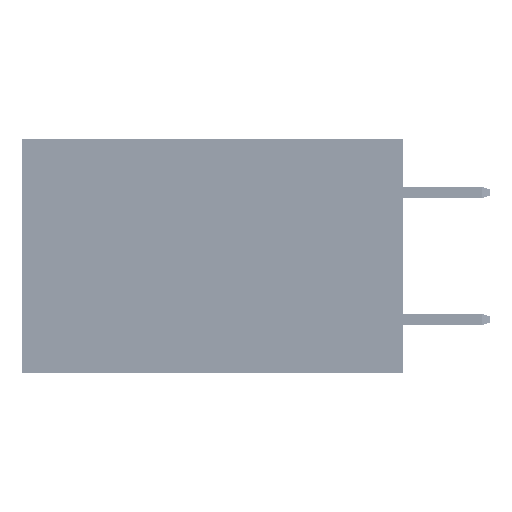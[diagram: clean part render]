
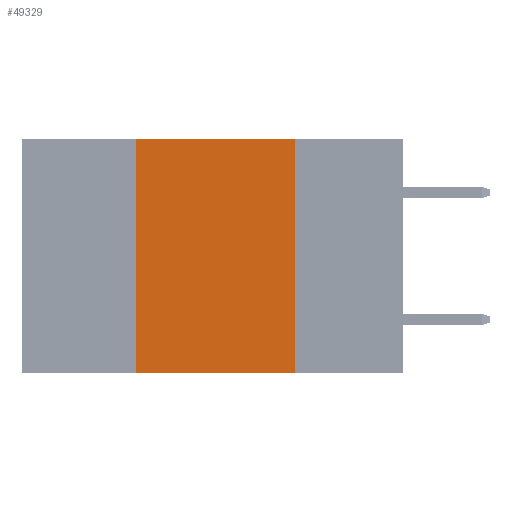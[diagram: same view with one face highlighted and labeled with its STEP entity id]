
A CAD part, left-side view. The second image highlights one B-rep face of the part: STEP entity #49329.
In plain terms, the highlighted planar face has unit normal (-1, 0, 0).
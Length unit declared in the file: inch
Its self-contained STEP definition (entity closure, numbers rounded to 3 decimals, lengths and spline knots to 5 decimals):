
#8373 = CARTESIAN_POINT ( 'NONE',  ( 0., 0.42, -0.37 ) ) ;
#9885 = ORIENTED_EDGE ( 'NONE', *, *, #15686, .F. ) ;
#10452 = DIRECTION ( 'NONE',  ( 0., 0., -1. ) ) ;
#10727 = VECTOR ( 'NONE', #41330, 39.37008 ) ;
#10737 = VERTEX_POINT ( 'NONE', #44114 ) ;
#11090 = VECTOR ( 'NONE', #43198, 39.37008 ) ;
#11476 = LINE ( 'NONE', #27892, #10727 ) ;
#12933 = PLANE ( 'NONE',  #31094 ) ;
#13321 = EDGE_LOOP ( 'NONE', ( #42781, #47987, #9885, #37089 ) ) ;
#15686 = EDGE_CURVE ( 'NONE', #40103, #10737, #46551, .T. ) ;
#16985 = CARTESIAN_POINT ( 'NONE',  ( 0., 0.6, 0. ) ) ;
#18684 = LINE ( 'NONE', #46978, #11090 ) ;
#22291 = DIRECTION ( 'NONE',  ( 0., 0., 1. ) ) ;
#22766 = CARTESIAN_POINT ( 'NONE',  ( 0., 0.17, 0. ) ) ;
#23977 = DIRECTION ( 'NONE',  ( 1., 0., 0. ) ) ;
#24784 = FACE_OUTER_BOUND ( 'NONE', #13321, .T. ) ;
#27892 = CARTESIAN_POINT ( 'NONE',  ( 0., 0.6, 0. ) ) ;
#28918 = EDGE_CURVE ( 'NONE', #40103, #43686, #18684, .T. ) ;
#30377 = CARTESIAN_POINT ( 'NONE',  ( 0., 0.42, 0. ) ) ;
#31094 = AXIS2_PLACEMENT_3D ( 'NONE', #16985, #23977, #48785 ) ;
#34374 = CARTESIAN_POINT ( 'NONE',  ( 0., 0.17, -0.37 ) ) ;
#37089 = ORIENTED_EDGE ( 'NONE', *, *, #28918, .T. ) ;
#37757 = EDGE_CURVE ( 'NONE', #10737, #52507, #11476, .T. ) ;
#37998 = VECTOR ( 'NONE', #22291, 39.37008 ) ;
#39527 = CARTESIAN_POINT ( 'NONE',  ( 0., 0.17, 0. ) ) ;
#40103 = VERTEX_POINT ( 'NONE', #8373 ) ;
#41330 = DIRECTION ( 'NONE',  ( 0., -1., 0. ) ) ;
#42781 = ORIENTED_EDGE ( 'NONE', *, *, #48281, .F. ) ;
#43198 = DIRECTION ( 'NONE',  ( 0., -1., 0. ) ) ;
#43589 = LINE ( 'NONE', #39527, #49992 ) ;
#43686 = VERTEX_POINT ( 'NONE', #34374 ) ;
#44114 = CARTESIAN_POINT ( 'NONE',  ( 0., 0.42, 0. ) ) ;
#46551 = LINE ( 'NONE', #30377, #37998 ) ;
#46978 = CARTESIAN_POINT ( 'NONE',  ( 0., 0.6, -0.37 ) ) ;
#47987 = ORIENTED_EDGE ( 'NONE', *, *, #37757, .F. ) ;
#48281 = EDGE_CURVE ( 'NONE', #52507, #43686, #43589, .T. ) ;
#48785 = DIRECTION ( 'NONE',  ( 0., 0., -1. ) ) ;
#49329 = ADVANCED_FACE ( 'NONE', ( #24784 ), #12933, .F. ) ;
#49992 = VECTOR ( 'NONE', #10452, 39.37008 ) ;
#52507 = VERTEX_POINT ( 'NONE', #22766 ) ;
